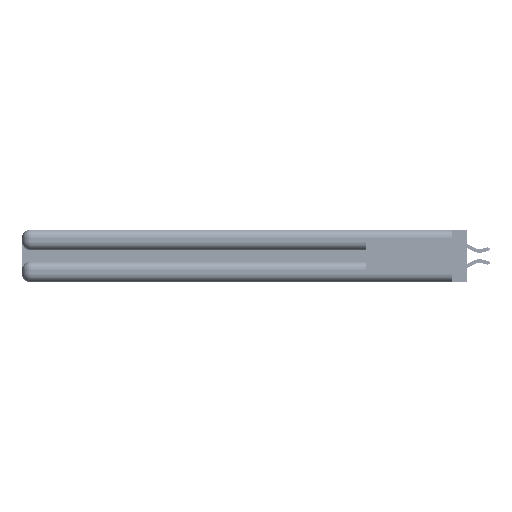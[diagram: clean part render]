
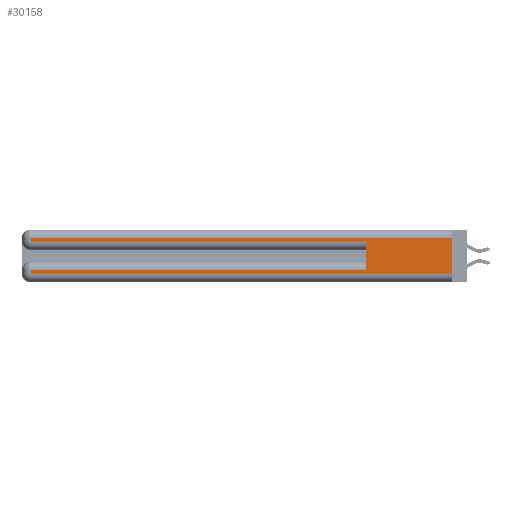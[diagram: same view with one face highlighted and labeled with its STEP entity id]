
A CAD part, left-side view. The second image highlights one B-rep face of the part: STEP entity #30158.
In plain terms, the highlighted planar face has unit normal (-1, 0, 0).
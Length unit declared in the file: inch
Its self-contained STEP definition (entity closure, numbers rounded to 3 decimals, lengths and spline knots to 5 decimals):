
#2119 = LINE ( 'NONE', #33031, #33896 ) ;
#2180 = LINE ( 'NONE', #34498, #22217 ) ;
#4418 = VERTEX_POINT ( 'NONE', #32527 ) ;
#5219 = VECTOR ( 'NONE', #41947, 39.37008 ) ;
#5728 = EDGE_CURVE ( 'NONE', #23780, #6841, #27275, .T. ) ;
#6841 = VERTEX_POINT ( 'NONE', #32247 ) ;
#8868 = EDGE_CURVE ( 'NONE', #19851, #6841, #46166, .T. ) ;
#11339 = ORIENTED_EDGE ( 'NONE', *, *, #12007, .T. ) ;
#11461 = VERTEX_POINT ( 'NONE', #16176 ) ;
#12007 = EDGE_CURVE ( 'NONE', #19799, #4418, #24784, .T. ) ;
#14569 = CARTESIAN_POINT ( 'NONE',  ( 0., 2.94, 0.37 ) ) ;
#15109 = DIRECTION ( 'NONE',  ( 0., 0., -1. ) ) ;
#16176 = CARTESIAN_POINT ( 'NONE',  ( 0., 2.94, 0.085 ) ) ;
#16230 = ORIENTED_EDGE ( 'NONE', *, *, #38924, .T. ) ;
#17056 = DIRECTION ( 'NONE',  ( 1., 0., 0. ) ) ;
#18587 = VECTOR ( 'NONE', #15109, 39.37008 ) ;
#19799 = VERTEX_POINT ( 'NONE', #42929 ) ;
#19851 = VERTEX_POINT ( 'NONE', #28835 ) ;
#20883 = LINE ( 'NONE', #26535, #5219 ) ;
#20910 = PLANE ( 'NONE',  #47377 ) ;
#22217 = VECTOR ( 'NONE', #46314, 39.37008 ) ;
#22300 = ORIENTED_EDGE ( 'NONE', *, *, #8868, .T. ) ;
#22369 = CARTESIAN_POINT ( 'NONE',  ( 0., 0.6, 0.285 ) ) ;
#23780 = VERTEX_POINT ( 'NONE', #24324 ) ;
#24324 = CARTESIAN_POINT ( 'NONE',  ( 0., 0., 0.31 ) ) ;
#24784 = LINE ( 'NONE', #14569, #32832 ) ;
#24949 = DIRECTION ( 'NONE',  ( 0., -1., 0. ) ) ;
#25053 = DIRECTION ( 'NONE',  ( 0., 0., -1. ) ) ;
#25959 = FACE_OUTER_BOUND ( 'NONE', #43303, .T. ) ;
#26531 = VERTEX_POINT ( 'NONE', #22369 ) ;
#26535 = CARTESIAN_POINT ( 'NONE',  ( 0., 0., 0.085 ) ) ;
#27275 = LINE ( 'NONE', #35038, #18587 ) ;
#28835 = CARTESIAN_POINT ( 'NONE',  ( 0., 2.94, 0.06 ) ) ;
#29790 = ORIENTED_EDGE ( 'NONE', *, *, #32725, .T. ) ;
#30158 = ADVANCED_FACE ( 'NONE', ( #25959 ), #20910, .F. ) ;
#31096 = VECTOR ( 'NONE', #47210, 39.37008 ) ;
#32247 = CARTESIAN_POINT ( 'NONE',  ( 0., 0., 0.06 ) ) ;
#32527 = CARTESIAN_POINT ( 'NONE',  ( 0., 2.94, 0.285 ) ) ;
#32725 = EDGE_CURVE ( 'NONE', #11461, #19851, #2180, .T. ) ;
#32832 = VECTOR ( 'NONE', #46479, 39.37008 ) ;
#33031 = CARTESIAN_POINT ( 'NONE',  ( 0., 0.6, 0.145 ) ) ;
#33896 = VECTOR ( 'NONE', #37181, 39.37008 ) ;
#34137 = VERTEX_POINT ( 'NONE', #43563 ) ;
#34498 = CARTESIAN_POINT ( 'NONE',  ( 0., 2.94, 0.37 ) ) ;
#35038 = CARTESIAN_POINT ( 'NONE',  ( 0., 0., 0.37 ) ) ;
#35600 = VECTOR ( 'NONE', #51111, 39.37008 ) ;
#35835 = EDGE_CURVE ( 'NONE', #34137, #11461, #20883, .T. ) ;
#37181 = DIRECTION ( 'NONE',  ( 0., 0., 1. ) ) ;
#38924 = EDGE_CURVE ( 'NONE', #4418, #26531, #49160, .T. ) ;
#39454 = CARTESIAN_POINT ( 'NONE',  ( 0., 0., 0.06 ) ) ;
#40063 = ORIENTED_EDGE ( 'NONE', *, *, #5728, .F. ) ;
#40803 = CARTESIAN_POINT ( 'NONE',  ( 0., 0., 0.37 ) ) ;
#41055 = CARTESIAN_POINT ( 'NONE',  ( 0., 0., 0.285 ) ) ;
#41442 = EDGE_CURVE ( 'NONE', #34137, #26531, #2119, .T. ) ;
#41609 = LINE ( 'NONE', #43218, #31096 ) ;
#41947 = DIRECTION ( 'NONE',  ( 0., 1., 0. ) ) ;
#42929 = CARTESIAN_POINT ( 'NONE',  ( 0., 2.94, 0.31 ) ) ;
#43218 = CARTESIAN_POINT ( 'NONE',  ( 0., 0., 0.31 ) ) ;
#43303 = EDGE_LOOP ( 'NONE', ( #40063, #46362, #11339, #16230, #51130, #44386, #29790, #22300 ) ) ;
#43563 = CARTESIAN_POINT ( 'NONE',  ( 0., 0.6, 0.085 ) ) ;
#44386 = ORIENTED_EDGE ( 'NONE', *, *, #35835, .T. ) ;
#46166 = LINE ( 'NONE', #39454, #35600 ) ;
#46314 = DIRECTION ( 'NONE',  ( 0., 0., -1. ) ) ;
#46362 = ORIENTED_EDGE ( 'NONE', *, *, #50406, .T. ) ;
#46479 = DIRECTION ( 'NONE',  ( 0., 0., -1. ) ) ;
#46648 = VECTOR ( 'NONE', #24949, 39.37008 ) ;
#47210 = DIRECTION ( 'NONE',  ( 0., 1., 0. ) ) ;
#47377 = AXIS2_PLACEMENT_3D ( 'NONE', #40803, #17056, #25053 ) ;
#49160 = LINE ( 'NONE', #41055, #46648 ) ;
#50406 = EDGE_CURVE ( 'NONE', #23780, #19799, #41609, .T. ) ;
#51111 = DIRECTION ( 'NONE',  ( 0., -1., 0. ) ) ;
#51130 = ORIENTED_EDGE ( 'NONE', *, *, #41442, .F. ) ;
